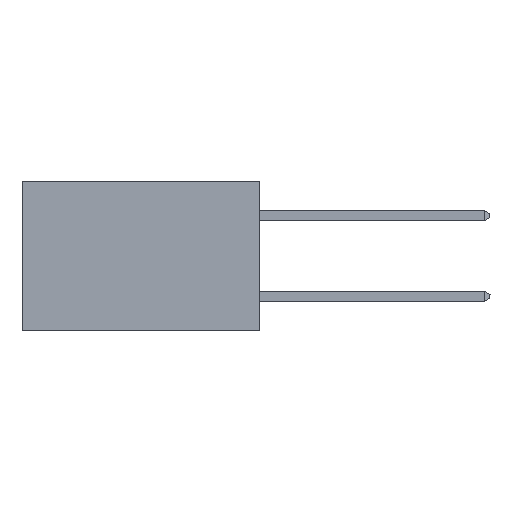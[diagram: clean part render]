
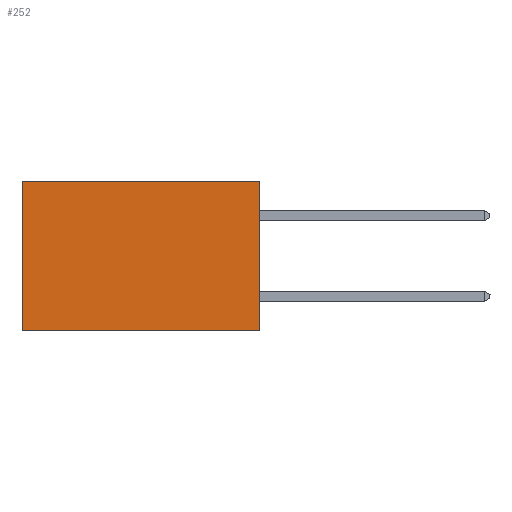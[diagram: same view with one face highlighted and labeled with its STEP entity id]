
A CAD part, left-side view. The second image highlights one B-rep face of the part: STEP entity #252.
In plain terms, the highlighted planar face has unit normal (-1, 0, 0).
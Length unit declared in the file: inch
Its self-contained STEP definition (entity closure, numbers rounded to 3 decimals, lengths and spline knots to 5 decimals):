
#223 = EDGE_LOOP ( 'NONE', ( #1133, #1157, #1308, #1367 ) ) ;
#252 = ADVANCED_FACE ( 'NONE', ( #1484 ), #5075, .F. ) ;
#277 = VECTOR ( 'NONE', #5043, 39.37008 ) ;
#634 = VERTEX_POINT ( 'NONE', #8454 ) ;
#831 = DIRECTION ( 'NONE',  ( 0., 0., -1. ) ) ;
#877 = CARTESIAN_POINT ( 'NONE',  ( 0.277, 0.59, -0.37 ) ) ;
#1069 = VECTOR ( 'NONE', #3109, 39.37008 ) ;
#1133 = ORIENTED_EDGE ( 'NONE', *, *, #2530, .T. ) ;
#1157 = ORIENTED_EDGE ( 'NONE', *, *, #1518, .F. ) ;
#1308 = ORIENTED_EDGE ( 'NONE', *, *, #1496, .F. ) ;
#1367 = ORIENTED_EDGE ( 'NONE', *, *, #3457, .T. ) ;
#1484 = FACE_OUTER_BOUND ( 'NONE', #223, .T. ) ;
#1496 = EDGE_CURVE ( 'NONE', #634, #8277, #6940, .T. ) ;
#1518 = EDGE_CURVE ( 'NONE', #8277, #7604, #9865, .T. ) ;
#1526 = AXIS2_PLACEMENT_3D ( 'NONE', #2222, #5421, #5383 ) ;
#2222 = CARTESIAN_POINT ( 'NONE',  ( 0.277, 0., -0.37 ) ) ;
#2530 = EDGE_CURVE ( 'NONE', #8900, #7604, #9727, .T. ) ;
#3109 = DIRECTION ( 'NONE',  ( 0., 1., 0. ) ) ;
#3160 = CARTESIAN_POINT ( 'NONE',  ( 0.277, 0.59, -0.37 ) ) ;
#3457 = EDGE_CURVE ( 'NONE', #634, #8900, #5851, .T. ) ;
#4163 = VECTOR ( 'NONE', #831, 39.37008 ) ;
#4438 = CARTESIAN_POINT ( 'NONE',  ( 0.277, 0., -0.37 ) ) ;
#4511 = CARTESIAN_POINT ( 'NONE',  ( 0.277, 0., -0.37 ) ) ;
#5043 = DIRECTION ( 'NONE',  ( 0., 1., 0. ) ) ;
#5075 = PLANE ( 'NONE',  #1526 ) ;
#5383 = DIRECTION ( 'NONE',  ( 0., 0., -1. ) ) ;
#5421 = DIRECTION ( 'NONE',  ( 1., 0., 0. ) ) ;
#5583 = CARTESIAN_POINT ( 'NONE',  ( 0.277, 0., 0. ) ) ;
#5851 = LINE ( 'NONE', #5583, #1069 ) ;
#6141 = DIRECTION ( 'NONE',  ( 0., 0., -1. ) ) ;
#6403 = CARTESIAN_POINT ( 'NONE',  ( 0.277, 0., -0.37 ) ) ;
#6940 = LINE ( 'NONE', #6403, #8740 ) ;
#7604 = VERTEX_POINT ( 'NONE', #3160 ) ;
#8277 = VERTEX_POINT ( 'NONE', #4511 ) ;
#8454 = CARTESIAN_POINT ( 'NONE',  ( 0.277, 0., 0. ) ) ;
#8740 = VECTOR ( 'NONE', #6141, 39.37008 ) ;
#8900 = VERTEX_POINT ( 'NONE', #9785 ) ;
#9727 = LINE ( 'NONE', #877, #4163 ) ;
#9785 = CARTESIAN_POINT ( 'NONE',  ( 0.277, 0.59, 0. ) ) ;
#9865 = LINE ( 'NONE', #4438, #277 ) ;
